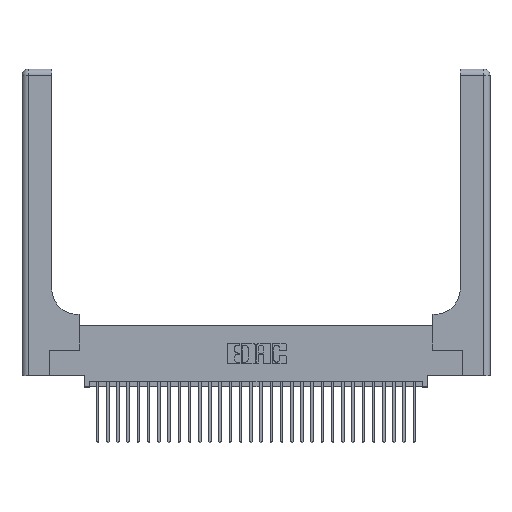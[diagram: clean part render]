
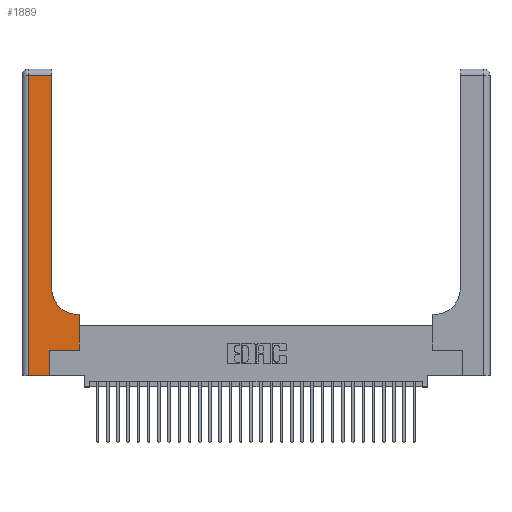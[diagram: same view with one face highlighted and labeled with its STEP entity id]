
A CAD part, top view. The second image highlights one B-rep face of the part: STEP entity #1889.
In plain terms, the highlighted planar face has unit normal (0, 0, 1).
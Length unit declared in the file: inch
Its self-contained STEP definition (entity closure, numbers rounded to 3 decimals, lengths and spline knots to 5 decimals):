
#404 = LINE ( 'NONE', #18590, #17795 ) ;
#837 = CARTESIAN_POINT ( 'NONE',  ( 0., 0., 0.37 ) ) ;
#913 = CARTESIAN_POINT ( 'NONE',  ( 0., 3., 0.37 ) ) ;
#1098 = CARTESIAN_POINT ( 'NONE',  ( 0.2915, 2.94, 0.37 ) ) ;
#1883 = CARTESIAN_POINT ( 'NONE',  ( 0.269, 0.25, 0.37 ) ) ;
#1889 = ADVANCED_FACE ( 'NONE', ( #2040 ), #5897, .F. ) ;
#2040 = FACE_OUTER_BOUND ( 'NONE', #29185, .T. ) ;
#2330 = VECTOR ( 'NONE', #13988, 39.37008 ) ;
#2364 = CARTESIAN_POINT ( 'NONE',  ( 0.5585, 0.25, 0.37 ) ) ;
#2802 = VERTEX_POINT ( 'NONE', #1098 ) ;
#2872 = EDGE_CURVE ( 'NONE', #26372, #9409, #404, .T. ) ;
#3784 = VERTEX_POINT ( 'NONE', #2364 ) ;
#4055 = VECTOR ( 'NONE', #27807, 39.37008 ) ;
#4172 = ORIENTED_EDGE ( 'NONE', *, *, #21589, .T. ) ;
#4230 = EDGE_CURVE ( 'NONE', #2802, #10224, #13920, .T. ) ;
#4698 = CIRCLE ( 'NONE', #31199, 0.25 ) ;
#5191 = VECTOR ( 'NONE', #28112, 39.37008 ) ;
#5371 = CARTESIAN_POINT ( 'NONE',  ( 0.06, 0., 0.37 ) ) ;
#5684 = DIRECTION ( 'NONE',  ( 0., 0., -1. ) ) ;
#5897 = PLANE ( 'NONE',  #11825 ) ;
#5999 = ORIENTED_EDGE ( 'NONE', *, *, #7065, .T. ) ;
#6845 = LINE ( 'NONE', #12980, #12673 ) ;
#7065 = EDGE_CURVE ( 'NONE', #19724, #26372, #17959, .T. ) ;
#7607 = VECTOR ( 'NONE', #19517, 39.37008 ) ;
#7733 = VERTEX_POINT ( 'NONE', #22001 ) ;
#8298 = CARTESIAN_POINT ( 'NONE',  ( 0.5585, 0.6, 0.37 ) ) ;
#8385 = LINE ( 'NONE', #17041, #7607 ) ;
#8390 = DIRECTION ( 'NONE',  ( 0., 0., -1. ) ) ;
#9068 = DIRECTION ( 'NONE',  ( 0., -1., 0. ) ) ;
#9192 = ORIENTED_EDGE ( 'NONE', *, *, #2872, .T. ) ;
#9409 = VERTEX_POINT ( 'NONE', #1883 ) ;
#10224 = VERTEX_POINT ( 'NONE', #19747 ) ;
#10876 = CARTESIAN_POINT ( 'NONE',  ( 0.2915, 0.6, 0.37 ) ) ;
#11229 = EDGE_CURVE ( 'NONE', #19472, #2802, #12962, .T. ) ;
#11425 = CARTESIAN_POINT ( 'NONE',  ( 0.2915, 0.85, 0.37 ) ) ;
#11471 = EDGE_CURVE ( 'NONE', #19307, #7733, #31264, .T. ) ;
#11825 = AXIS2_PLACEMENT_3D ( 'NONE', #913, #8390, #25538 ) ;
#12673 = VECTOR ( 'NONE', #20407, 39.37008 ) ;
#12962 = LINE ( 'NONE', #17595, #25199 ) ;
#12980 = CARTESIAN_POINT ( 'NONE',  ( 0.5585, 0.25, 0.37 ) ) ;
#13920 = LINE ( 'NONE', #28601, #2330 ) ;
#13988 = DIRECTION ( 'NONE',  ( -1., 0., 0. ) ) ;
#16275 = ORIENTED_EDGE ( 'NONE', *, *, #4230, .T. ) ;
#16469 = ORIENTED_EDGE ( 'NONE', *, *, #30992, .T. ) ;
#17041 = CARTESIAN_POINT ( 'NONE',  ( 0.269, 0.25, 0.37 ) ) ;
#17595 = CARTESIAN_POINT ( 'NONE',  ( 0.2915, 3., 0.37 ) ) ;
#17795 = VECTOR ( 'NONE', #21054, 39.37008 ) ;
#17959 = LINE ( 'NONE', #837, #4055 ) ;
#18590 = CARTESIAN_POINT ( 'NONE',  ( 0.269, 0., 0.37 ) ) ;
#18873 = CARTESIAN_POINT ( 'NONE',  ( 0.06, 3., 0.37 ) ) ;
#19307 = VERTEX_POINT ( 'NONE', #8298 ) ;
#19472 = VERTEX_POINT ( 'NONE', #11425 ) ;
#19517 = DIRECTION ( 'NONE',  ( 1., 0., 0. ) ) ;
#19724 = VERTEX_POINT ( 'NONE', #5371 ) ;
#19747 = CARTESIAN_POINT ( 'NONE',  ( 0.06, 2.94, 0.37 ) ) ;
#20077 = DIRECTION ( 'NONE',  ( 0., 1., 0. ) ) ;
#20156 = ORIENTED_EDGE ( 'NONE', *, *, #21189, .T. ) ;
#20407 = DIRECTION ( 'NONE',  ( 0., 1., 0. ) ) ;
#20470 = CARTESIAN_POINT ( 'NONE',  ( 0.5415, 0.85, 0.37 ) ) ;
#21054 = DIRECTION ( 'NONE',  ( 0., 1., 0. ) ) ;
#21189 = EDGE_CURVE ( 'NONE', #3784, #19307, #6845, .T. ) ;
#21279 = CARTESIAN_POINT ( 'NONE',  ( 0.269, 0., 0.37 ) ) ;
#21589 = EDGE_CURVE ( 'NONE', #9409, #3784, #8385, .T. ) ;
#21979 = ORIENTED_EDGE ( 'NONE', *, *, #11229, .T. ) ;
#22001 = CARTESIAN_POINT ( 'NONE',  ( 0.5415, 0.6, 0.37 ) ) ;
#22838 = LINE ( 'NONE', #18873, #24582 ) ;
#22893 = DIRECTION ( 'NONE',  ( 1., 0., 0. ) ) ;
#24582 = VECTOR ( 'NONE', #9068, 39.37008 ) ;
#24740 = ORIENTED_EDGE ( 'NONE', *, *, #26894, .T. ) ;
#25199 = VECTOR ( 'NONE', #20077, 39.37008 ) ;
#25538 = DIRECTION ( 'NONE',  ( -1., 0., 0. ) ) ;
#26372 = VERTEX_POINT ( 'NONE', #21279 ) ;
#26711 = ORIENTED_EDGE ( 'NONE', *, *, #11471, .T. ) ;
#26894 = EDGE_CURVE ( 'NONE', #10224, #19724, #22838, .T. ) ;
#27807 = DIRECTION ( 'NONE',  ( 1., 0., 0. ) ) ;
#28112 = DIRECTION ( 'NONE',  ( -1., 0., 0. ) ) ;
#28601 = CARTESIAN_POINT ( 'NONE',  ( 0., 2.94, 0.37 ) ) ;
#29185 = EDGE_LOOP ( 'NONE', ( #21979, #16275, #24740, #5999, #9192, #4172, #20156, #26711, #16469 ) ) ;
#30992 = EDGE_CURVE ( 'NONE', #7733, #19472, #4698, .T. ) ;
#31199 = AXIS2_PLACEMENT_3D ( 'NONE', #20470, #5684, #22893 ) ;
#31264 = LINE ( 'NONE', #10876, #5191 ) ;
